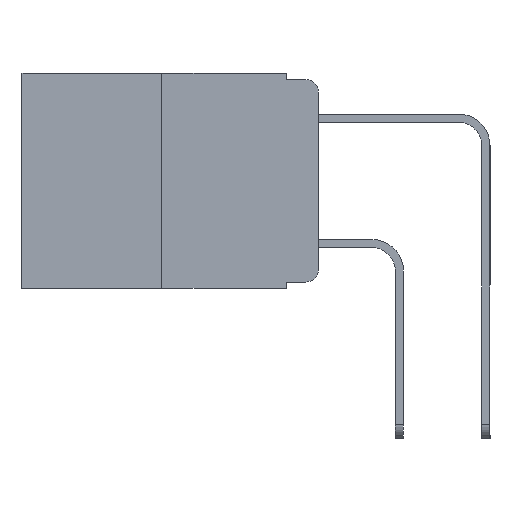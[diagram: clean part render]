
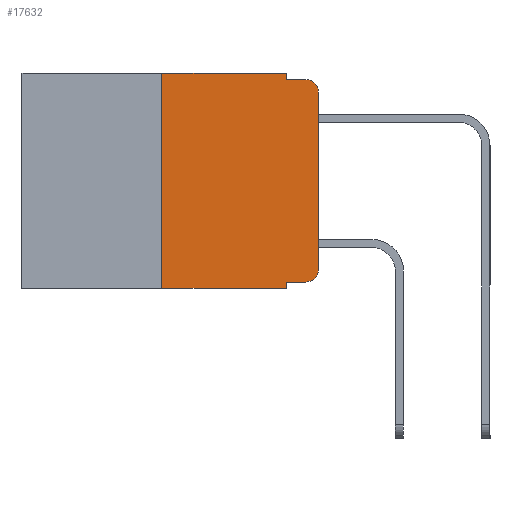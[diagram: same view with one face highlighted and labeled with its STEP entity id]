
A CAD part, left-side view. The second image highlights one B-rep face of the part: STEP entity #17632.
In plain terms, the highlighted planar face has unit normal (-1, 0, 0).
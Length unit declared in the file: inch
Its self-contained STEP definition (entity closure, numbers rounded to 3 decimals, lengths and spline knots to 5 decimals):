
#281 = LINE ( 'NONE', #11933, #21049 ) ;
#438 = CARTESIAN_POINT ( 'NONE',  ( 0., 0.02, -0.01 ) ) ;
#746 = VERTEX_POINT ( 'NONE', #16782 ) ;
#793 = LINE ( 'NONE', #986, #13571 ) ;
#986 = CARTESIAN_POINT ( 'NONE',  ( 0., 0.051, 0. ) ) ;
#1085 = VECTOR ( 'NONE', #16057, 39.37008 ) ;
#1322 = ORIENTED_EDGE ( 'NONE', *, *, #13836, .T. ) ;
#1390 = FACE_OUTER_BOUND ( 'NONE', #16958, .T. ) ;
#1840 = LINE ( 'NONE', #13725, #14889 ) ;
#1957 = DIRECTION ( 'NONE',  ( -1., 0., 0. ) ) ;
#2101 = DIRECTION ( 'NONE',  ( 0., -1., 0. ) ) ;
#3161 = LINE ( 'NONE', #15591, #7112 ) ;
#3253 = LINE ( 'NONE', #19855, #20324 ) ;
#3739 = AXIS2_PLACEMENT_3D ( 'NONE', #11906, #1957, #13474 ) ;
#3811 = CARTESIAN_POINT ( 'NONE',  ( 0., 0., -0.313 ) ) ;
#3913 = ORIENTED_EDGE ( 'NONE', *, *, #12908, .F. ) ;
#3924 = CARTESIAN_POINT ( 'NONE',  ( 0., 0.25, 0. ) ) ;
#4090 = DIRECTION ( 'NONE',  ( 0., -1., 0. ) ) ;
#4441 = ORIENTED_EDGE ( 'NONE', *, *, #19859, .T. ) ;
#4526 = VECTOR ( 'NONE', #15928, 39.37008 ) ;
#4710 = CIRCLE ( 'NONE', #3739, 0.02 ) ;
#4958 = ORIENTED_EDGE ( 'NONE', *, *, #17088, .F. ) ;
#5469 = VERTEX_POINT ( 'NONE', #8685 ) ;
#5609 = VERTEX_POINT ( 'NONE', #438 ) ;
#5772 = CARTESIAN_POINT ( 'NONE',  ( 0., 0.051, -0.01 ) ) ;
#6196 = EDGE_CURVE ( 'NONE', #20650, #5609, #18025, .T. ) ;
#6346 = VERTEX_POINT ( 'NONE', #7690 ) ;
#6606 = VERTEX_POINT ( 'NONE', #16112 ) ;
#6617 = PLANE ( 'NONE',  #15218 ) ;
#7112 = VECTOR ( 'NONE', #20358, 39.37008 ) ;
#7247 = DIRECTION ( 'NONE',  ( 0., -1., 0. ) ) ;
#7638 = VERTEX_POINT ( 'NONE', #16822 ) ;
#7690 = CARTESIAN_POINT ( 'NONE',  ( 0., 0.051, 0. ) ) ;
#8239 = DIRECTION ( 'NONE',  ( 0., 0., -1. ) ) ;
#8242 = EDGE_CURVE ( 'NONE', #5469, #746, #16902, .T. ) ;
#8685 = CARTESIAN_POINT ( 'NONE',  ( 0., 0.051, -0.333 ) ) ;
#8934 = CARTESIAN_POINT ( 'NONE',  ( 0., 0.02, -0.03 ) ) ;
#9190 = VERTEX_POINT ( 'NONE', #5772 ) ;
#9571 = LINE ( 'NONE', #14450, #1085 ) ;
#9754 = CARTESIAN_POINT ( 'NONE',  ( 0., 0.473, 0. ) ) ;
#10007 = ORIENTED_EDGE ( 'NONE', *, *, #15380, .F. ) ;
#10544 = DIRECTION ( 'NONE',  ( 0., 0., -1. ) ) ;
#11036 = ORIENTED_EDGE ( 'NONE', *, *, #16434, .F. ) ;
#11537 = VERTEX_POINT ( 'NONE', #3924 ) ;
#11647 = CARTESIAN_POINT ( 'NONE',  ( 0., 0.051, -0.333 ) ) ;
#11906 = CARTESIAN_POINT ( 'NONE',  ( 0., 0.02, -0.313 ) ) ;
#11933 = CARTESIAN_POINT ( 'NONE',  ( 0., 0.473, 0. ) ) ;
#12081 = CARTESIAN_POINT ( 'NONE',  ( 0., 0., -0.03 ) ) ;
#12908 = EDGE_CURVE ( 'NONE', #6606, #11537, #9571, .T. ) ;
#13241 = ORIENTED_EDGE ( 'NONE', *, *, #17219, .T. ) ;
#13474 = DIRECTION ( 'NONE',  ( 0., 0., -1. ) ) ;
#13571 = VECTOR ( 'NONE', #15754, 39.37008 ) ;
#13578 = LINE ( 'NONE', #17509, #4526 ) ;
#13725 = CARTESIAN_POINT ( 'NONE',  ( 0., 0.051, -0.01 ) ) ;
#13836 = EDGE_CURVE ( 'NONE', #746, #13881, #4710, .T. ) ;
#13881 = VERTEX_POINT ( 'NONE', #3811 ) ;
#14450 = CARTESIAN_POINT ( 'NONE',  ( 0., 0.25, 0. ) ) ;
#14889 = VECTOR ( 'NONE', #4090, 39.37008 ) ;
#15218 = AXIS2_PLACEMENT_3D ( 'NONE', #9754, #17694, #8239 ) ;
#15380 = EDGE_CURVE ( 'NONE', #9190, #5609, #1840, .T. ) ;
#15591 = CARTESIAN_POINT ( 'NONE',  ( 0., 0.051, 0. ) ) ;
#15702 = ORIENTED_EDGE ( 'NONE', *, *, #16138, .F. ) ;
#15754 = DIRECTION ( 'NONE',  ( 0., 0., -1. ) ) ;
#15923 = VECTOR ( 'NONE', #16296, 39.37008 ) ;
#15928 = DIRECTION ( 'NONE',  ( 0., 0., 1. ) ) ;
#16057 = DIRECTION ( 'NONE',  ( 0., 0., 1. ) ) ;
#16112 = CARTESIAN_POINT ( 'NONE',  ( 0., 0.25, -0.343 ) ) ;
#16138 = EDGE_CURVE ( 'NONE', #11537, #6346, #281, .T. ) ;
#16296 = DIRECTION ( 'NONE',  ( 0., -1., 0. ) ) ;
#16434 = EDGE_CURVE ( 'NONE', #6346, #9190, #793, .T. ) ;
#16782 = CARTESIAN_POINT ( 'NONE',  ( 0., 0.02, -0.333 ) ) ;
#16822 = CARTESIAN_POINT ( 'NONE',  ( 0., 0.051, -0.343 ) ) ;
#16902 = LINE ( 'NONE', #11647, #15923 ) ;
#16958 = EDGE_LOOP ( 'NONE', ( #13241, #17907, #10007, #11036, #15702, #3913, #4441, #4958, #17666, #1322 ) ) ;
#17088 = EDGE_CURVE ( 'NONE', #5469, #7638, #3161, .T. ) ;
#17219 = EDGE_CURVE ( 'NONE', #13881, #20650, #13578, .T. ) ;
#17509 = CARTESIAN_POINT ( 'NONE',  ( 0., 0., 0. ) ) ;
#17632 = ADVANCED_FACE ( 'NONE', ( #1390 ), #6617, .F. ) ;
#17666 = ORIENTED_EDGE ( 'NONE', *, *, #8242, .T. ) ;
#17694 = DIRECTION ( 'NONE',  ( 1., 0., 0. ) ) ;
#17907 = ORIENTED_EDGE ( 'NONE', *, *, #6196, .T. ) ;
#18025 = CIRCLE ( 'NONE', #20673, 0.02 ) ;
#19855 = CARTESIAN_POINT ( 'NONE',  ( 0., 0.473, -0.343 ) ) ;
#19859 = EDGE_CURVE ( 'NONE', #6606, #7638, #3253, .T. ) ;
#19992 = DIRECTION ( 'NONE',  ( -1., 0., 0. ) ) ;
#20324 = VECTOR ( 'NONE', #2101, 39.37008 ) ;
#20358 = DIRECTION ( 'NONE',  ( 0., 0., -1. ) ) ;
#20650 = VERTEX_POINT ( 'NONE', #12081 ) ;
#20673 = AXIS2_PLACEMENT_3D ( 'NONE', #8934, #19992, #10544 ) ;
#21049 = VECTOR ( 'NONE', #7247, 39.37008 ) ;
